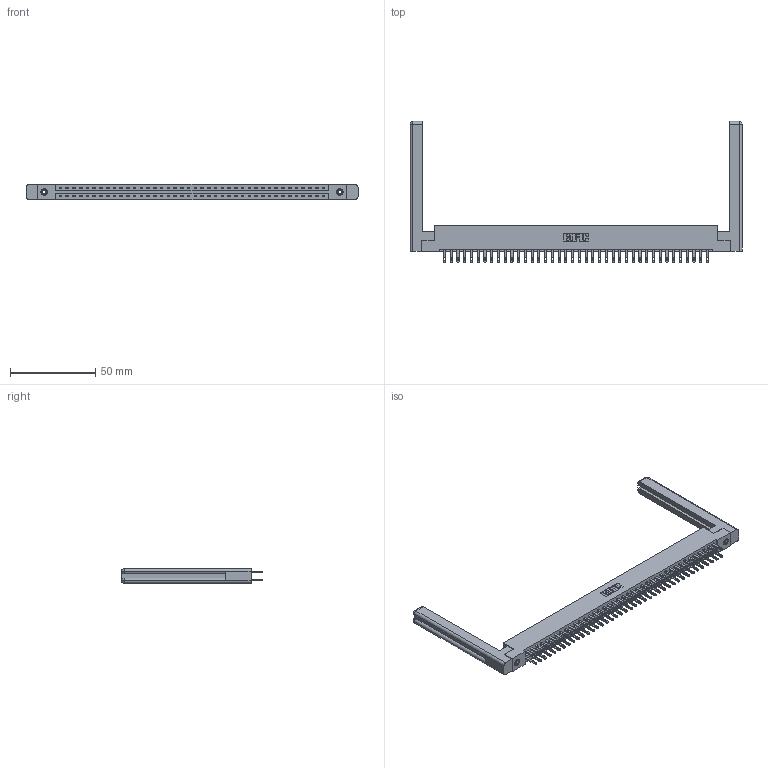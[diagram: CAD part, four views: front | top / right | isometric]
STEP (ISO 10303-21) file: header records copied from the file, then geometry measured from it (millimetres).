
FILE_DESCRIPTION (( 'STEP AP203' ), '1' );
FILE_NAME ('337-080-500-258.STEP', '2019-10-10T11:54:09', ( '' ), ( '' ), 'SwSTEP 2.0', 'SolidWorks 2016', '' );
FILE_SCHEMA (( 'CONFIG_CONTROL_DESIGN' ));
Length unit declared in the file: inch
Products named in the file (5): 337-080-500-258; 307-220-058; 337 Part_Flush Mounting Lugs - 0.156 Dia-TI; 345-292-001_345-293-100; 345-250-001_345-250-001-102
Assembly tree (85 placements, depth 2):
  337-080-500-258
    337 Part_Flush Mounting Lugs - 0.156 Dia-TI
    345-292-001_345-293-100  x80
    345-250-001_345-250-001-102  x2
    307-220-058  x2
Bounding box: 195.12 x 82.94 x 9.4 mm (x, y, z)
Volume: 27923.8 mm3; surface area: 29408.4 mm2
Topology: 85 solids, 85 shells, 4256 faces, 12905 edges, 8590 vertices
Faces by surface type: plane 2714, cylinder 1518, cone 12, torus 12
Entity records: 33836 total; most frequent: CARTESIAN_POINT 5709, ORIENTED_EDGE 5584, DIRECTION 4876, EDGE_CURVE 2792, LINE 2612, VECTOR 2612, VERTEX_POINT 1854, AXIS2_PLACEMENT_3D 1132
